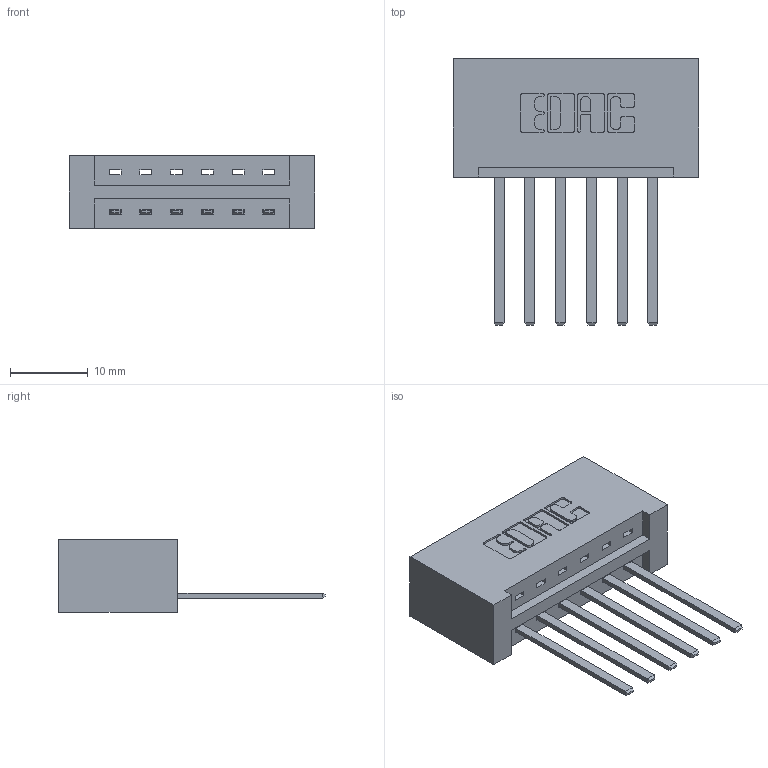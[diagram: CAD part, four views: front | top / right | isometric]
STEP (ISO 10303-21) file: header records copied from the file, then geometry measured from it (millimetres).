
FILE_DESCRIPTION (( 'STEP AP203' ), '1' );
FILE_NAME ('337-006-544-101.STEP', '2019-09-27T17:17:53', ( '' ), ( '' ), 'SwSTEP 2.0', 'SolidWorks 2016', '' );
FILE_SCHEMA (( 'CONFIG_CONTROL_DESIGN' ));
Length unit declared in the file: inch
Products named in the file (3): 337-006-544-101; 337 Part_No Mounting Lugs; 345-292-001_345-293-144
Assembly tree (7 placements, depth 2):
  337-006-544-101
    337 Part_No Mounting Lugs
    345-292-001_345-293-144  x6
Bounding box: 31.65 x 34.3 x 9.4 mm (x, y, z)
Volume: 3647 mm3; surface area: 3778.9 mm2
Topology: 7 solids, 7 shells, 442 faces, 1307 edges, 862 vertices
Faces by surface type: plane 318, cylinder 124
Entity records: 8655 total; most frequent: CARTESIAN_POINT 1512, ORIENTED_EDGE 1454, DIRECTION 1335, EDGE_CURVE 727, VECTOR 611, LINE 611, VERTEX_POINT 482, AXIS2_PLACEMENT_3D 362
